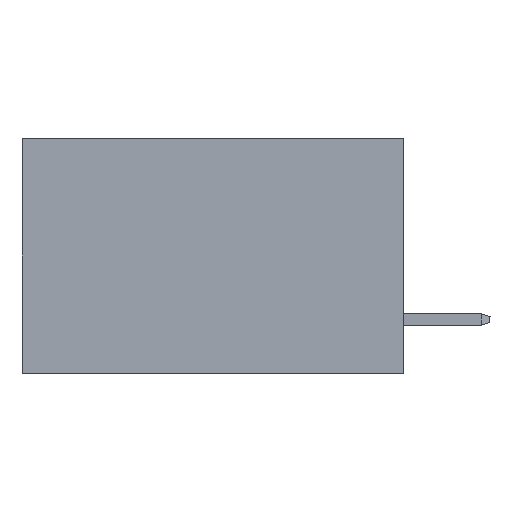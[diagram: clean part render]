
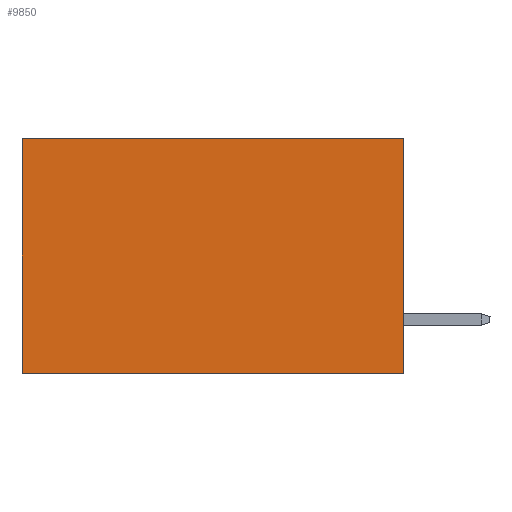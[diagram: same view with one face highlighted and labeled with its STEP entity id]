
A CAD part, left-side view. The second image highlights one B-rep face of the part: STEP entity #9850.
In plain terms, the highlighted planar face has unit normal (-1, 0, 0).
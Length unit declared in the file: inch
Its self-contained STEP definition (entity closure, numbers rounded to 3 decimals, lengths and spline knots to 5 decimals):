
#2889 = EDGE_CURVE ( 'NONE', #24922, #6989, #3075, .T. ) ;
#3075 = LINE ( 'NONE', #7377, #22091 ) ;
#4807 = CARTESIAN_POINT ( 'NONE',  ( 0.2875, 0.6, 0. ) ) ;
#5755 = LINE ( 'NONE', #26692, #22756 ) ;
#6989 = VERTEX_POINT ( 'NONE', #4807 ) ;
#7377 = CARTESIAN_POINT ( 'NONE',  ( 0.2875, 0., 0. ) ) ;
#8023 = DIRECTION ( 'NONE',  ( 0., 0., -1. ) ) ;
#8277 = VECTOR ( 'NONE', #14891, 39.37008 ) ;
#9850 = ADVANCED_FACE ( 'NONE', ( #14459 ), #21201, .F. ) ;
#10379 = VERTEX_POINT ( 'NONE', #15859 ) ;
#10570 = CARTESIAN_POINT ( 'NONE',  ( 0.2875, 0., 0. ) ) ;
#11180 = EDGE_CURVE ( 'NONE', #24922, #16679, #19952, .T. ) ;
#11908 = ORIENTED_EDGE ( 'NONE', *, *, #19549, .F. ) ;
#12696 = ORIENTED_EDGE ( 'NONE', *, *, #11180, .F. ) ;
#13538 = AXIS2_PLACEMENT_3D ( 'NONE', #27695, #21344, #8023 ) ;
#14459 = FACE_OUTER_BOUND ( 'NONE', #22306, .T. ) ;
#14891 = DIRECTION ( 'NONE',  ( 0., 1., 0. ) ) ;
#15414 = ORIENTED_EDGE ( 'NONE', *, *, #27190, .T. ) ;
#15859 = CARTESIAN_POINT ( 'NONE',  ( 0.2875, 0.6, -0.37 ) ) ;
#16679 = VERTEX_POINT ( 'NONE', #26602 ) ;
#18066 = VECTOR ( 'NONE', #24050, 39.37008 ) ;
#19549 = EDGE_CURVE ( 'NONE', #16679, #10379, #21051, .T. ) ;
#19952 = LINE ( 'NONE', #22047, #18066 ) ;
#20765 = CARTESIAN_POINT ( 'NONE',  ( 0.2875, 0., -0.37 ) ) ;
#21051 = LINE ( 'NONE', #20765, #8277 ) ;
#21201 = PLANE ( 'NONE',  #13538 ) ;
#21344 = DIRECTION ( 'NONE',  ( 1., 0., 0. ) ) ;
#21509 = ORIENTED_EDGE ( 'NONE', *, *, #2889, .T. ) ;
#22047 = CARTESIAN_POINT ( 'NONE',  ( 0.2875, 0., 0. ) ) ;
#22091 = VECTOR ( 'NONE', #26764, 39.37008 ) ;
#22306 = EDGE_LOOP ( 'NONE', ( #15414, #11908, #12696, #21509 ) ) ;
#22756 = VECTOR ( 'NONE', #26974, 39.37008 ) ;
#24050 = DIRECTION ( 'NONE',  ( 0., 0., -1. ) ) ;
#24922 = VERTEX_POINT ( 'NONE', #10570 ) ;
#26602 = CARTESIAN_POINT ( 'NONE',  ( 0.2875, 0., -0.37 ) ) ;
#26692 = CARTESIAN_POINT ( 'NONE',  ( 0.2875, 0.6, 0. ) ) ;
#26764 = DIRECTION ( 'NONE',  ( 0., 1., 0. ) ) ;
#26974 = DIRECTION ( 'NONE',  ( 0., 0., -1. ) ) ;
#27190 = EDGE_CURVE ( 'NONE', #6989, #10379, #5755, .T. ) ;
#27695 = CARTESIAN_POINT ( 'NONE',  ( 0.2875, 0., 0. ) ) ;
